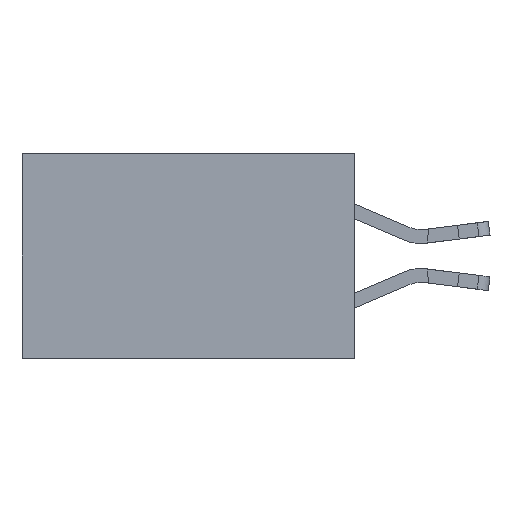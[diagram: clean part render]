
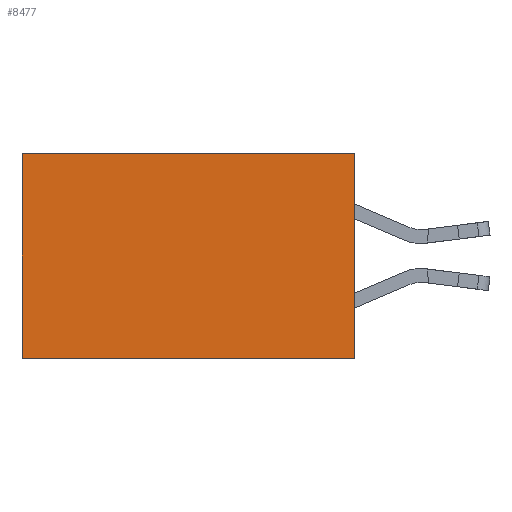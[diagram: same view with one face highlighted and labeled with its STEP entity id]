
A CAD part, left-side view. The second image highlights one B-rep face of the part: STEP entity #8477.
In plain terms, the highlighted planar face has unit normal (-1, 0, 0).
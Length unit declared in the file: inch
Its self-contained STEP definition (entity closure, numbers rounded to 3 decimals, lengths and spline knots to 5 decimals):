
#1202 = ORIENTED_EDGE ( 'NONE', *, *, #9644, .F. ) ;
#3073 = VECTOR ( 'NONE', #8083, 39.37008 ) ;
#3277 = CARTESIAN_POINT ( 'NONE',  ( 0.298, 0., 0. ) ) ;
#3569 = CARTESIAN_POINT ( 'NONE',  ( 0.298, 0., 0. ) ) ;
#3722 = VERTEX_POINT ( 'NONE', #3277 ) ;
#4098 = ORIENTED_EDGE ( 'NONE', *, *, #7708, .T. ) ;
#4128 = DIRECTION ( 'NONE',  ( 0., 0., -1. ) ) ;
#4251 = LINE ( 'NONE', #13612, #10008 ) ;
#4254 = DIRECTION ( 'NONE',  ( 0., 1., 0. ) ) ;
#4305 = DIRECTION ( 'NONE',  ( 1., 0., 0. ) ) ;
#4455 = DIRECTION ( 'NONE',  ( 0., 1., 0. ) ) ;
#4566 = PLANE ( 'NONE',  #9962 ) ;
#5792 = CARTESIAN_POINT ( 'NONE',  ( 0.298, 0.6, 0. ) ) ;
#6411 = VECTOR ( 'NONE', #12289, 39.37008 ) ;
#6492 = LINE ( 'NONE', #11684, #10202 ) ;
#6799 = LINE ( 'NONE', #7223, #6411 ) ;
#7223 = CARTESIAN_POINT ( 'NONE',  ( 0.298, 0., 0. ) ) ;
#7708 = EDGE_CURVE ( 'NONE', #12980, #14035, #13299, .T. ) ;
#7798 = FACE_OUTER_BOUND ( 'NONE', #8345, .T. ) ;
#7864 = CARTESIAN_POINT ( 'NONE',  ( 0.298, 0.6, -0.37 ) ) ;
#8083 = DIRECTION ( 'NONE',  ( 0., 0., -1. ) ) ;
#8345 = EDGE_LOOP ( 'NONE', ( #4098, #1202, #11988, #12164 ) ) ;
#8477 = ADVANCED_FACE ( 'NONE', ( #7798 ), #4566, .F. ) ;
#9644 = EDGE_CURVE ( 'NONE', #12156, #14035, #4251, .T. ) ;
#9962 = AXIS2_PLACEMENT_3D ( 'NONE', #3569, #4305, #4128 ) ;
#10008 = VECTOR ( 'NONE', #4455, 39.37008 ) ;
#10202 = VECTOR ( 'NONE', #4254, 39.37008 ) ;
#10429 = EDGE_CURVE ( 'NONE', #3722, #12980, #6492, .T. ) ;
#11453 = CARTESIAN_POINT ( 'NONE',  ( 0.298, 0., -0.37 ) ) ;
#11684 = CARTESIAN_POINT ( 'NONE',  ( 0.298, 0., 0. ) ) ;
#11988 = ORIENTED_EDGE ( 'NONE', *, *, #15298, .F. ) ;
#12156 = VERTEX_POINT ( 'NONE', #11453 ) ;
#12164 = ORIENTED_EDGE ( 'NONE', *, *, #10429, .T. ) ;
#12289 = DIRECTION ( 'NONE',  ( 0., 0., -1. ) ) ;
#12980 = VERTEX_POINT ( 'NONE', #5792 ) ;
#13299 = LINE ( 'NONE', #14064, #3073 ) ;
#13612 = CARTESIAN_POINT ( 'NONE',  ( 0.298, 0., -0.37 ) ) ;
#14035 = VERTEX_POINT ( 'NONE', #7864 ) ;
#14064 = CARTESIAN_POINT ( 'NONE',  ( 0.298, 0.6, 0. ) ) ;
#15298 = EDGE_CURVE ( 'NONE', #3722, #12156, #6799, .T. ) ;
